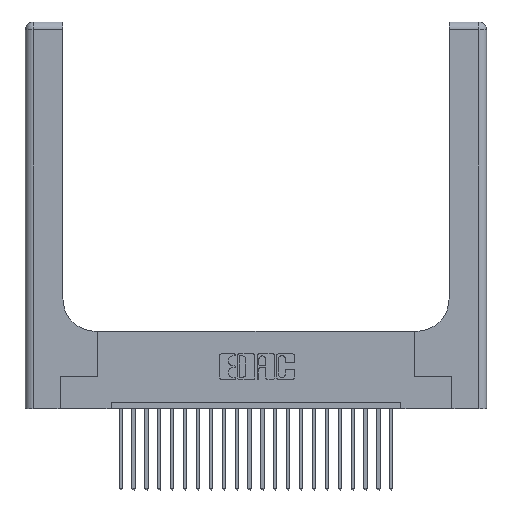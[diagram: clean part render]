
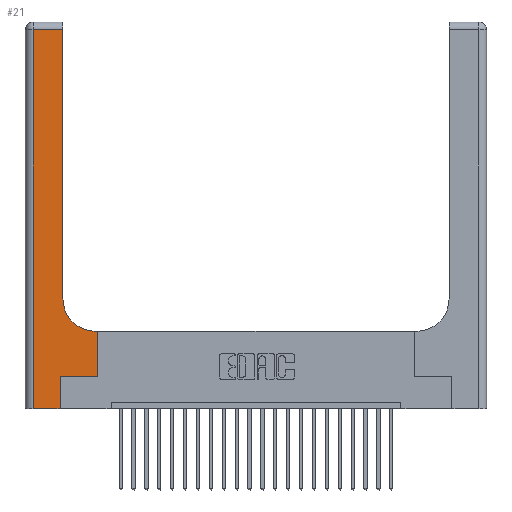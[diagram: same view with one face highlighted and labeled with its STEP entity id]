
A CAD part, top view. The second image highlights one B-rep face of the part: STEP entity #21.
In plain terms, the highlighted planar face has unit normal (0, 0, 1).
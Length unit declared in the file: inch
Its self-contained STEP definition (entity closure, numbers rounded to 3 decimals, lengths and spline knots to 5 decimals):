
#21 = ADVANCED_FACE ( 'NONE', ( #15660 ), #21817, .F. ) ;
#60 = ORIENTED_EDGE ( 'NONE', *, *, #9657, .T. ) ;
#501 = DIRECTION ( 'NONE',  ( 0., 0., -1. ) ) ;
#523 = VERTEX_POINT ( 'NONE', #15758 ) ;
#1062 = DIRECTION ( 'NONE',  ( 0., 0., -1. ) ) ;
#2622 = CARTESIAN_POINT ( 'NONE',  ( 0., 3., 0.37 ) ) ;
#2717 = VECTOR ( 'NONE', #3061, 39.37008 ) ;
#2851 = ORIENTED_EDGE ( 'NONE', *, *, #16486, .T. ) ;
#3061 = DIRECTION ( 'NONE',  ( 1., 0., 0. ) ) ;
#3297 = DIRECTION ( 'NONE',  ( -1., 0., 0. ) ) ;
#3653 = VECTOR ( 'NONE', #19781, 39.37008 ) ;
#3733 = ORIENTED_EDGE ( 'NONE', *, *, #13284, .T. ) ;
#4080 = CIRCLE ( 'NONE', #7517, 0.25 ) ;
#4154 = CARTESIAN_POINT ( 'NONE',  ( 0.5415, 0.85, 0.37 ) ) ;
#4194 = CARTESIAN_POINT ( 'NONE',  ( 0.5585, 0.25, 0.37 ) ) ;
#4442 = VECTOR ( 'NONE', #7267, 39.37008 ) ;
#4581 = ORIENTED_EDGE ( 'NONE', *, *, #9750, .T. ) ;
#4744 = VERTEX_POINT ( 'NONE', #10285 ) ;
#4919 = CARTESIAN_POINT ( 'NONE',  ( 0.2915, 0.6, 0.37 ) ) ;
#5422 = ORIENTED_EDGE ( 'NONE', *, *, #24342, .T. ) ;
#5484 = VECTOR ( 'NONE', #17380, 39.37008 ) ;
#6589 = LINE ( 'NONE', #10962, #12195 ) ;
#6648 = ORIENTED_EDGE ( 'NONE', *, *, #20683, .T. ) ;
#7183 = VECTOR ( 'NONE', #11127, 39.37008 ) ;
#7267 = DIRECTION ( 'NONE',  ( 1., 0., 0. ) ) ;
#7517 = AXIS2_PLACEMENT_3D ( 'NONE', #4154, #501, #19348 ) ;
#7900 = VERTEX_POINT ( 'NONE', #18306 ) ;
#8284 = VERTEX_POINT ( 'NONE', #16476 ) ;
#9217 = DIRECTION ( 'NONE',  ( 0., 1., 0. ) ) ;
#9406 = DIRECTION ( 'NONE',  ( 0., 1., 0. ) ) ;
#9657 = EDGE_CURVE ( 'NONE', #8284, #4744, #11589, .T. ) ;
#9716 = VECTOR ( 'NONE', #9217, 39.37008 ) ;
#9750 = EDGE_CURVE ( 'NONE', #19277, #23881, #6589, .T. ) ;
#9774 = ORIENTED_EDGE ( 'NONE', *, *, #9960, .T. ) ;
#9960 = EDGE_CURVE ( 'NONE', #16557, #8284, #13631, .T. ) ;
#10007 = EDGE_CURVE ( 'NONE', #7900, #18816, #15418, .T. ) ;
#10285 = CARTESIAN_POINT ( 'NONE',  ( 0.06, 0., 0.37 ) ) ;
#10925 = LINE ( 'NONE', #16488, #2717 ) ;
#10962 = CARTESIAN_POINT ( 'NONE',  ( 0.269, 0., 0.37 ) ) ;
#11127 = DIRECTION ( 'NONE',  ( 0., -1., 0. ) ) ;
#11470 = LINE ( 'NONE', #18594, #4442 ) ;
#11589 = LINE ( 'NONE', #18941, #7183 ) ;
#12195 = VECTOR ( 'NONE', #9406, 39.37008 ) ;
#13284 = EDGE_CURVE ( 'NONE', #15591, #7900, #21800, .T. ) ;
#13413 = EDGE_LOOP ( 'NONE', ( #23848, #9774, #60, #2851, #4581, #6648, #3733, #21143, #5422 ) ) ;
#13631 = LINE ( 'NONE', #21948, #3653 ) ;
#15418 = LINE ( 'NONE', #4919, #24298 ) ;
#15591 = VERTEX_POINT ( 'NONE', #15869 ) ;
#15660 = FACE_OUTER_BOUND ( 'NONE', #13413, .T. ) ;
#15758 = CARTESIAN_POINT ( 'NONE',  ( 0.2915, 0.85, 0.37 ) ) ;
#15869 = CARTESIAN_POINT ( 'NONE',  ( 0.5585, 0.25, 0.37 ) ) ;
#15949 = EDGE_CURVE ( 'NONE', #523, #16557, #23971, .T. ) ;
#16052 = DIRECTION ( 'NONE',  ( -1., 0., 0. ) ) ;
#16311 = CARTESIAN_POINT ( 'NONE',  ( 0.269, 0.25, 0.37 ) ) ;
#16476 = CARTESIAN_POINT ( 'NONE',  ( 0.06, 2.94, 0.37 ) ) ;
#16486 = EDGE_CURVE ( 'NONE', #4744, #19277, #10925, .T. ) ;
#16488 = CARTESIAN_POINT ( 'NONE',  ( 0., 0., 0.37 ) ) ;
#16557 = VERTEX_POINT ( 'NONE', #23779 ) ;
#16753 = CARTESIAN_POINT ( 'NONE',  ( 0.2915, 3., 0.37 ) ) ;
#17380 = DIRECTION ( 'NONE',  ( 0., 1., 0. ) ) ;
#17567 = CARTESIAN_POINT ( 'NONE',  ( 0.269, 0., 0.37 ) ) ;
#18306 = CARTESIAN_POINT ( 'NONE',  ( 0.5585, 0.6, 0.37 ) ) ;
#18594 = CARTESIAN_POINT ( 'NONE',  ( 0.269, 0.25, 0.37 ) ) ;
#18816 = VERTEX_POINT ( 'NONE', #21691 ) ;
#18941 = CARTESIAN_POINT ( 'NONE',  ( 0.06, 3., 0.37 ) ) ;
#19277 = VERTEX_POINT ( 'NONE', #17567 ) ;
#19348 = DIRECTION ( 'NONE',  ( 1., 0., 0. ) ) ;
#19781 = DIRECTION ( 'NONE',  ( -1., 0., 0. ) ) ;
#20683 = EDGE_CURVE ( 'NONE', #23881, #15591, #11470, .T. ) ;
#21143 = ORIENTED_EDGE ( 'NONE', *, *, #10007, .T. ) ;
#21691 = CARTESIAN_POINT ( 'NONE',  ( 0.5415, 0.6, 0.37 ) ) ;
#21800 = LINE ( 'NONE', #4194, #5484 ) ;
#21817 = PLANE ( 'NONE',  #22785 ) ;
#21948 = CARTESIAN_POINT ( 'NONE',  ( 0., 2.94, 0.37 ) ) ;
#22785 = AXIS2_PLACEMENT_3D ( 'NONE', #2622, #1062, #3297 ) ;
#23779 = CARTESIAN_POINT ( 'NONE',  ( 0.2915, 2.94, 0.37 ) ) ;
#23848 = ORIENTED_EDGE ( 'NONE', *, *, #15949, .T. ) ;
#23881 = VERTEX_POINT ( 'NONE', #16311 ) ;
#23971 = LINE ( 'NONE', #16753, #9716 ) ;
#24298 = VECTOR ( 'NONE', #16052, 39.37008 ) ;
#24342 = EDGE_CURVE ( 'NONE', #18816, #523, #4080, .T. ) ;
